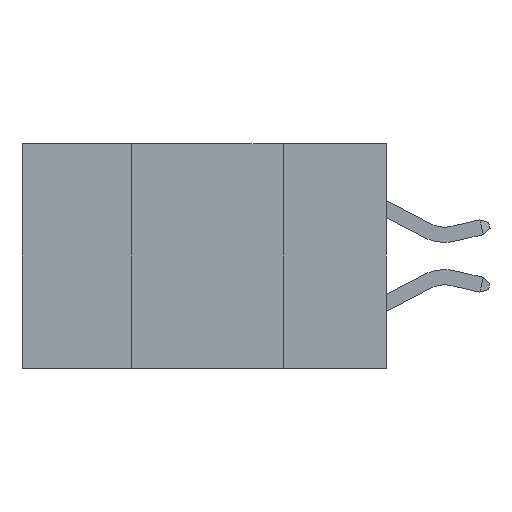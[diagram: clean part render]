
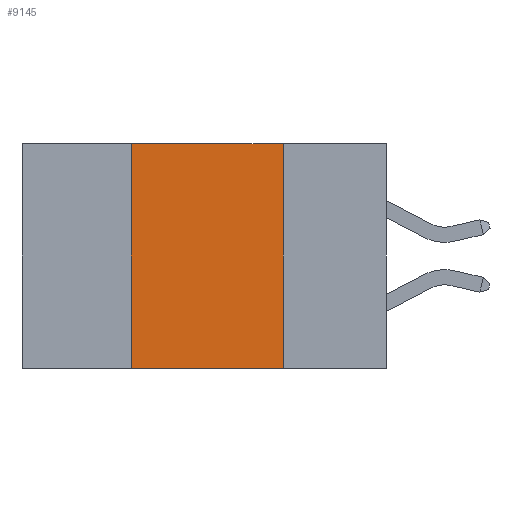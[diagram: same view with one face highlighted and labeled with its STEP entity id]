
A CAD part, left-side view. The second image highlights one B-rep face of the part: STEP entity #9145.
In plain terms, the highlighted planar face has unit normal (-1, 0, 0).
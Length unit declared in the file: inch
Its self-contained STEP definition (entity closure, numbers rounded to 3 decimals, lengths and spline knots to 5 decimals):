
#1206 = CARTESIAN_POINT ( 'NONE',  ( 0., 0.42, -0.37 ) ) ;
#1697 = CARTESIAN_POINT ( 'NONE',  ( 0., 0.6, 0. ) ) ;
#2097 = EDGE_CURVE ( 'NONE', #16844, #12806, #5859, .T. ) ;
#3167 = EDGE_CURVE ( 'NONE', #16844, #8399, #7065, .T. ) ;
#3298 = DIRECTION ( 'NONE',  ( 0., 0., -1. ) ) ;
#3927 = ORIENTED_EDGE ( 'NONE', *, *, #4276, .F. ) ;
#4116 = ORIENTED_EDGE ( 'NONE', *, *, #8671, .F. ) ;
#4208 = ORIENTED_EDGE ( 'NONE', *, *, #3167, .F. ) ;
#4230 = ORIENTED_EDGE ( 'NONE', *, *, #2097, .T. ) ;
#4276 = EDGE_CURVE ( 'NONE', #11936, #12806, #7542, .T. ) ;
#4538 = DIRECTION ( 'NONE',  ( 0., 0., 1. ) ) ;
#5859 = LINE ( 'NONE', #9920, #6373 ) ;
#5861 = CARTESIAN_POINT ( 'NONE',  ( 0., 0.17, -0.37 ) ) ;
#6267 = CARTESIAN_POINT ( 'NONE',  ( 0., 0.42, 0. ) ) ;
#6373 = VECTOR ( 'NONE', #17920, 39.37008 ) ;
#6582 = VECTOR ( 'NONE', #4538, 39.37008 ) ;
#7065 = LINE ( 'NONE', #6267, #6582 ) ;
#7278 = VECTOR ( 'NONE', #12940, 39.37008 ) ;
#7542 = LINE ( 'NONE', #19514, #15480 ) ;
#8399 = VERTEX_POINT ( 'NONE', #9168 ) ;
#8671 = EDGE_CURVE ( 'NONE', #8399, #11936, #12467, .T. ) ;
#8774 = FACE_OUTER_BOUND ( 'NONE', #13751, .T. ) ;
#9145 = ADVANCED_FACE ( 'NONE', ( #8774 ), #11300, .F. ) ;
#9168 = CARTESIAN_POINT ( 'NONE',  ( 0., 0.42, 0. ) ) ;
#9920 = CARTESIAN_POINT ( 'NONE',  ( 0., 0.6, -0.37 ) ) ;
#10348 = CARTESIAN_POINT ( 'NONE',  ( 0., 0.17, 0. ) ) ;
#11300 = PLANE ( 'NONE',  #18046 ) ;
#11936 = VERTEX_POINT ( 'NONE', #10348 ) ;
#12467 = LINE ( 'NONE', #14567, #7278 ) ;
#12806 = VERTEX_POINT ( 'NONE', #5861 ) ;
#12895 = DIRECTION ( 'NONE',  ( 1., 0., 0. ) ) ;
#12940 = DIRECTION ( 'NONE',  ( 0., -1., 0. ) ) ;
#13751 = EDGE_LOOP ( 'NONE', ( #3927, #4116, #4208, #4230 ) ) ;
#14567 = CARTESIAN_POINT ( 'NONE',  ( 0., 0.6, 0. ) ) ;
#15480 = VECTOR ( 'NONE', #17499, 39.37008 ) ;
#16844 = VERTEX_POINT ( 'NONE', #1206 ) ;
#17499 = DIRECTION ( 'NONE',  ( 0., 0., -1. ) ) ;
#17920 = DIRECTION ( 'NONE',  ( 0., -1., 0. ) ) ;
#18046 = AXIS2_PLACEMENT_3D ( 'NONE', #1697, #12895, #3298 ) ;
#19514 = CARTESIAN_POINT ( 'NONE',  ( 0., 0.17, 0. ) ) ;
